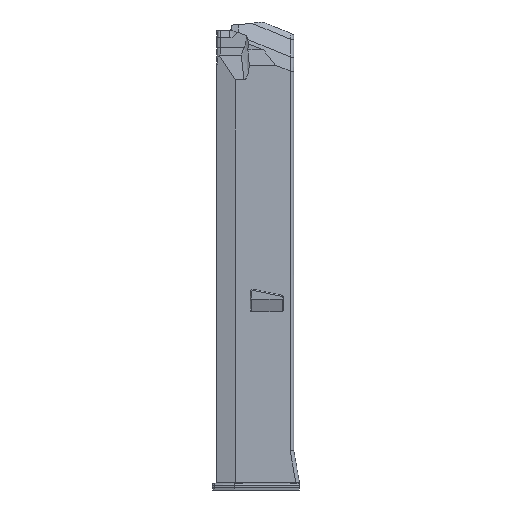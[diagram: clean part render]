
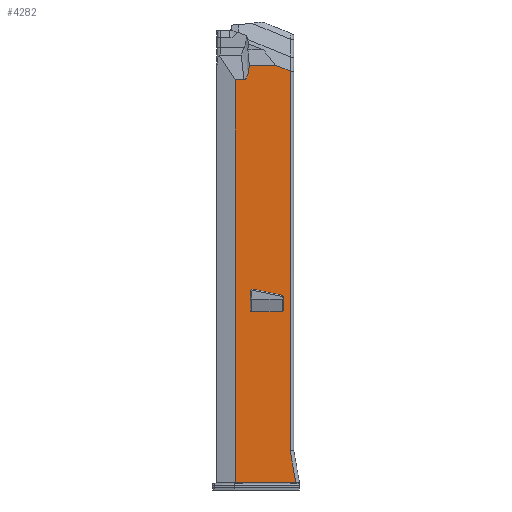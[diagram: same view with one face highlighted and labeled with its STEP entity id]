
A CAD part, left-side view. The second image highlights one B-rep face of the part: STEP entity #4282.
In plain terms, the highlighted planar face has unit normal (-1, 0, 0).
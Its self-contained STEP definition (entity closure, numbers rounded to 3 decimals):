
#99=FACE_BOUND('',#706,.T.);
#448=FACE_OUTER_BOUND('',#705,.T.);
#705=EDGE_LOOP('',(#3926,#3927,#3928,#3929,#3930,#3931,#3932,#3933));
#706=EDGE_LOOP('',(#3934,#3935,#3936,#3937,#3938,#3939,#3940,#3941));
#785=ELLIPSE('',#4462,1.005,1.);
#787=ELLIPSE('',#4465,1.005,1.);
#789=ELLIPSE('',#4468,1.463,0.503);
#793=ELLIPSE('',#4476,1.463,0.503);
#854=B_SPLINE_CURVE_WITH_KNOTS('',3,(#5596,#5597,#5598,#5599,#5600,#5601,
#5602,#5603,#5604,#5605,#5606,#5607,#5608),.UNSPECIFIED.,.F.,.F.,(4,3,3,
3,4),(0.44,0.612,0.907,1.091,
1.202),.UNSPECIFIED.);
#1008=LINE('',#5524,#1324);
#1015=LINE('',#5611,#1331);
#1115=LINE('',#6682,#1431);
#1120=LINE('',#6748,#1436);
#1125=LINE('',#6766,#1441);
#1193=LINE('',#8427,#1509);
#1196=LINE('',#8435,#1512);
#1201=LINE('',#8457,#1517);
#1204=LINE('',#8473,#1520);
#1292=LINE('',#10888,#1608);
#1313=LINE('',#11101,#1629);
#1324=VECTOR('',#4599,10.);
#1331=VECTOR('',#4612,10.043);
#1431=VECTOR('',#4850,10.05);
#1436=VECTOR('',#4869,10.002);
#1441=VECTOR('',#4882,10.);
#1509=VECTOR('',#5100,10.05);
#1512=VECTOR('',#5105,10.);
#1517=VECTOR('',#5116,10.048);
#1520=VECTOR('',#5125,10.);
#1608=VECTOR('',#5395,10.05);
#1629=VECTOR('',#5452,10.);
#1649=VERTEX_POINT('',#5518);
#1650=VERTEX_POINT('',#5523);
#1660=VERTEX_POINT('',#5591);
#1661=VERTEX_POINT('',#5610);
#1761=VERTEX_POINT('',#6607);
#1771=VERTEX_POINT('',#6681);
#1775=VERTEX_POINT('',#6746);
#1778=VERTEX_POINT('',#6765);
#1890=VERTEX_POINT('',#8423);
#1891=VERTEX_POINT('',#8425);
#1894=VERTEX_POINT('',#8432);
#1895=VERTEX_POINT('',#8434);
#1897=VERTEX_POINT('',#8449);
#1899=VERTEX_POINT('',#8455);
#1901=VERTEX_POINT('',#8466);
#1903=VERTEX_POINT('',#8471);
#2048=EDGE_CURVE('',#1650,#1649,#1008,.T.);
#2061=EDGE_CURVE('',#1660,#1649,#854,.F.);
#2062=EDGE_CURVE('',#1650,#1661,#1015,.T.);
#2225=EDGE_CURVE('',#1761,#1771,#1115,.T.);
#2237=EDGE_CURVE('',#1775,#1761,#1120,.T.);
#2243=EDGE_CURVE('',#1778,#1771,#1125,.T.);
#2408=EDGE_CURVE('',#1891,#1890,#1193,.T.);
#2411=EDGE_CURVE('',#1894,#1895,#1196,.T.);
#2415=EDGE_CURVE('',#1894,#1897,#785,.F.);
#2418=EDGE_CURVE('',#1899,#1897,#1201,.T.);
#2421=EDGE_CURVE('',#1899,#1901,#787,.F.);
#2423=EDGE_CURVE('',#1903,#1901,#1204,.T.);
#2426=EDGE_CURVE('',#1891,#1895,#789,.F.);
#2432=EDGE_CURVE('',#1903,#1890,#793,.F.);
#2637=EDGE_CURVE('',#1778,#1660,#1292,.T.);
#2665=EDGE_CURVE('',#1661,#1775,#1313,.T.);
#3926=ORIENTED_EDGE('',*,*,#2048,.T.);
#3927=ORIENTED_EDGE('',*,*,#2061,.F.);
#3928=ORIENTED_EDGE('',*,*,#2637,.F.);
#3929=ORIENTED_EDGE('',*,*,#2243,.T.);
#3930=ORIENTED_EDGE('',*,*,#2225,.F.);
#3931=ORIENTED_EDGE('',*,*,#2237,.F.);
#3932=ORIENTED_EDGE('',*,*,#2665,.F.);
#3933=ORIENTED_EDGE('',*,*,#2062,.F.);
#3934=ORIENTED_EDGE('',*,*,#2408,.F.);
#3935=ORIENTED_EDGE('',*,*,#2426,.T.);
#3936=ORIENTED_EDGE('',*,*,#2411,.F.);
#3937=ORIENTED_EDGE('',*,*,#2415,.T.);
#3938=ORIENTED_EDGE('',*,*,#2418,.F.);
#3939=ORIENTED_EDGE('',*,*,#2421,.T.);
#3940=ORIENTED_EDGE('',*,*,#2423,.F.);
#3941=ORIENTED_EDGE('',*,*,#2432,.T.);
#4039=PLANE('',#4576);
#4282=ADVANCED_FACE('',(#448,#99),#4039,.T.);
#4462=AXIS2_PLACEMENT_3D('',#8451,#5110,#5111);
#4465=AXIS2_PLACEMENT_3D('',#8468,#5120,#5121);
#4468=AXIS2_PLACEMENT_3D('',#8482,#5129,#5130);
#4476=AXIS2_PLACEMENT_3D('',#8664,#5145,#5146);
#4576=AXIS2_PLACEMENT_3D('',#11102,#5453,#5454);
#4599=DIRECTION('',(0.,1.,0.));
#4612=DIRECTION('',(0.,-0.925,-0.381));
#4850=DIRECTION('',(0.,1.,0.));
#4869=DIRECTION('',(0.,-0.177,-0.984));
#4882=DIRECTION('',(0.,0.,-1.));
#5100=DIRECTION('',(0.,-1.,0.));
#5105=DIRECTION('',(0.,0.,-1.));
#5110=DIRECTION('center_axis',(-1.,0.,0.));
#5111=DIRECTION('ref_axis',(0.,1.,0.));
#5116=DIRECTION('',(0.,0.98,0.198));
#5120=DIRECTION('center_axis',(-1.,0.,0.));
#5121=DIRECTION('ref_axis',(0.,1.,0.));
#5125=DIRECTION('',(0.,0.,1.));
#5129=DIRECTION('center_axis',(-1.,0.,0.));
#5130=DIRECTION('ref_axis',(0.,0.,
-1.));
#5145=DIRECTION('center_axis',(-1.,0.,0.));
#5146=DIRECTION('ref_axis',(0.,0.,-1.));
#5395=DIRECTION('',(0.,-1.,0.));
#5452=DIRECTION('',(0.,0.,-1.));
#5453=DIRECTION('center_axis',(-1.,0.,0.));
#5454=DIRECTION('ref_axis',(0.,0.,1.));
#5518=CARTESIAN_POINT('',(-10.605,2.488,125.254));
#5523=CARTESIAN_POINT('',(-10.605,-8.743,125.254));
#5524=CARTESIAN_POINT('',(-10.605,-7.106,125.254));
#5591=CARTESIAN_POINT('',(-10.605,4.794,118.95));
#5596=CARTESIAN_POINT('Ctrl Pts',(-10.605,2.488,125.254));
#5597=CARTESIAN_POINT('Ctrl Pts',(-10.605,2.551,124.671));
#5598=CARTESIAN_POINT('Ctrl Pts',(-10.605,2.625,124.084));
#5599=CARTESIAN_POINT('Ctrl Pts',(-10.605,2.721,123.473));
#5600=CARTESIAN_POINT('Ctrl Pts',(-10.605,2.885,122.43));
#5601=CARTESIAN_POINT('Ctrl Pts',(-10.605,3.107,121.378));
#5602=CARTESIAN_POINT('Ctrl Pts',(-10.605,3.411,120.551));
#5603=CARTESIAN_POINT('Ctrl Pts',(-10.605,3.6,120.035));
#5604=CARTESIAN_POINT('Ctrl Pts',(-10.605,3.808,119.598));
#5605=CARTESIAN_POINT('Ctrl Pts',(-10.605,4.115,119.28));
#5606=CARTESIAN_POINT('Ctrl Pts',(-10.605,4.301,119.089));
#5607=CARTESIAN_POINT('Ctrl Pts',(-10.605,4.534,118.95));
#5608=CARTESIAN_POINT('Ctrl Pts',(-10.605,4.794,118.95));
#5610=CARTESIAN_POINT('',(-10.605,-14.867,122.73));
#5611=CARTESIAN_POINT('',(-10.605,-32.651,115.4));
#6607=CARTESIAN_POINT('',(-10.605,-17.266,-52.3));
#6681=CARTESIAN_POINT('',(-10.605,8.6,-52.3));
#6682=CARTESIAN_POINT('',(-10.605,-8.214,-52.3));
#6746=CARTESIAN_POINT('',(-10.605,-14.867,-38.933));
#6748=CARTESIAN_POINT('',(-10.605,-16.431,-47.651));
#6765=CARTESIAN_POINT('',(-10.605,8.6,118.95));
#6766=CARTESIAN_POINT('',(-10.605,8.6,6.3));
#8423=CARTESIAN_POINT('',(-10.605,-11.532,20.2));
#8425=CARTESIAN_POINT('',(-10.605,1.533,20.2));
#8427=CARTESIAN_POINT('',(-10.605,-14.205,20.2));
#8432=CARTESIAN_POINT('',(-10.605,2.035,28.824));
#8434=CARTESIAN_POINT('',(-10.605,2.035,21.663));
#8435=CARTESIAN_POINT('',(-10.605,2.035,13.25));
#8449=CARTESIAN_POINT('',(-10.605,0.83,29.804));
#8451=CARTESIAN_POINT('Origin',(-10.605,1.03,28.824));
#8455=CARTESIAN_POINT('',(-10.605,-11.23,27.363));
#8457=CARTESIAN_POINT('',(-10.605,-9.135,27.787));
#8466=CARTESIAN_POINT('',(-10.605,-12.035,26.383));
#8468=CARTESIAN_POINT('Origin',(-10.605,-11.03,26.383));
#8471=CARTESIAN_POINT('',(-10.605,-12.035,21.663));
#8473=CARTESIAN_POINT('',(-10.605,-12.035,16.75));
#8482=CARTESIAN_POINT('Origin',(-10.605,1.533,21.663));
#8664=CARTESIAN_POINT('Origin',(-10.605,-11.532,21.663));
#10888=CARTESIAN_POINT('',(-10.605,-0.043,118.95));
#11101=CARTESIAN_POINT('',(-10.605,-14.867,-49.3));
#11102=CARTESIAN_POINT('Origin',(-10.605,-16.374,6.3));
